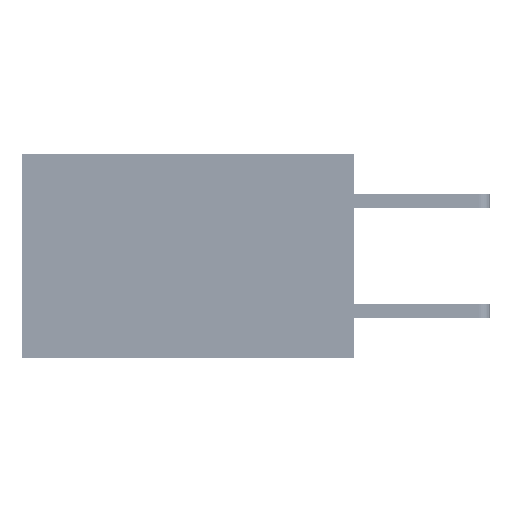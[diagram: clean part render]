
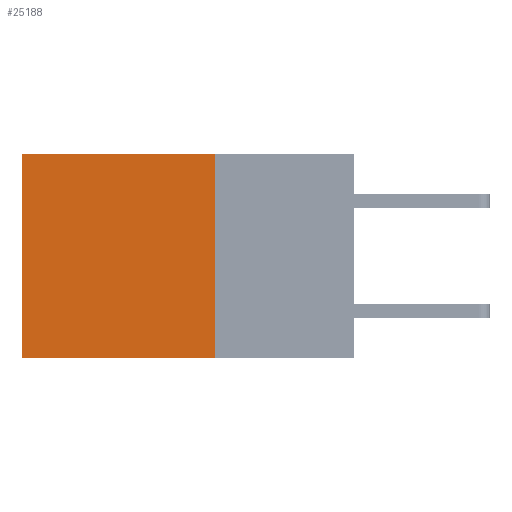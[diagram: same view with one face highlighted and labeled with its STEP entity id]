
A CAD part, left-side view. The second image highlights one B-rep face of the part: STEP entity #25188.
In plain terms, the highlighted planar face has unit normal (-1, 0, 0).
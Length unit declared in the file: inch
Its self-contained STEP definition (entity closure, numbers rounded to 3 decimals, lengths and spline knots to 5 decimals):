
#1695 = DIRECTION ( 'NONE',  ( 0., 1., 0. ) ) ;
#2542 = VERTEX_POINT ( 'NONE', #12695 ) ;
#2620 = AXIS2_PLACEMENT_3D ( 'NONE', #23223, #5068, #12479 ) ;
#5068 = DIRECTION ( 'NONE',  ( 1., 0., 0. ) ) ;
#5517 = LINE ( 'NONE', #20104, #5625 ) ;
#5625 = VECTOR ( 'NONE', #34702, 39.37008 ) ;
#6753 = EDGE_LOOP ( 'NONE', ( #38846, #31208, #15130, #32880 ) ) ;
#9839 = LINE ( 'NONE', #16293, #15713 ) ;
#10565 = EDGE_CURVE ( 'NONE', #2542, #46473, #35155, .T. ) ;
#10755 = LINE ( 'NONE', #43278, #37892 ) ;
#12479 = DIRECTION ( 'NONE',  ( 0., 0., -1. ) ) ;
#12555 = CARTESIAN_POINT ( 'NONE',  ( 0.2875, 0.25, 0. ) ) ;
#12695 = CARTESIAN_POINT ( 'NONE',  ( 0.2875, 0.25, -0.37 ) ) ;
#15130 = ORIENTED_EDGE ( 'NONE', *, *, #26478, .F. ) ;
#15713 = VECTOR ( 'NONE', #35189, 39.37008 ) ;
#16293 = CARTESIAN_POINT ( 'NONE',  ( 0.2875, 0.25, 0. ) ) ;
#18525 = CARTESIAN_POINT ( 'NONE',  ( 0.2875, 0.6, -0.37 ) ) ;
#20104 = CARTESIAN_POINT ( 'NONE',  ( 0.2875, 0.25, 0. ) ) ;
#20325 = CARTESIAN_POINT ( 'NONE',  ( 0.2875, 0.25, -0.37 ) ) ;
#21247 = EDGE_CURVE ( 'NONE', #44401, #46473, #10755, .T. ) ;
#22271 = EDGE_CURVE ( 'NONE', #35496, #44401, #5517, .T. ) ;
#23223 = CARTESIAN_POINT ( 'NONE',  ( 0.2875, 0.25, 0. ) ) ;
#23646 = CARTESIAN_POINT ( 'NONE',  ( 0.2875, 0.6, 0. ) ) ;
#25177 = VECTOR ( 'NONE', #1695, 39.37008 ) ;
#25188 = ADVANCED_FACE ( 'NONE', ( #45219 ), #38780, .F. ) ;
#26478 = EDGE_CURVE ( 'NONE', #35496, #2542, #9839, .T. ) ;
#31208 = ORIENTED_EDGE ( 'NONE', *, *, #10565, .F. ) ;
#32880 = ORIENTED_EDGE ( 'NONE', *, *, #22271, .T. ) ;
#34702 = DIRECTION ( 'NONE',  ( 0., 1., 0. ) ) ;
#35155 = LINE ( 'NONE', #20325, #25177 ) ;
#35189 = DIRECTION ( 'NONE',  ( 0., 0., -1. ) ) ;
#35496 = VERTEX_POINT ( 'NONE', #12555 ) ;
#36105 = DIRECTION ( 'NONE',  ( 0., 0., -1. ) ) ;
#37892 = VECTOR ( 'NONE', #36105, 39.37008 ) ;
#38780 = PLANE ( 'NONE',  #2620 ) ;
#38846 = ORIENTED_EDGE ( 'NONE', *, *, #21247, .T. ) ;
#43278 = CARTESIAN_POINT ( 'NONE',  ( 0.2875, 0.6, 0. ) ) ;
#44401 = VERTEX_POINT ( 'NONE', #23646 ) ;
#45219 = FACE_OUTER_BOUND ( 'NONE', #6753, .T. ) ;
#46473 = VERTEX_POINT ( 'NONE', #18525 ) ;
